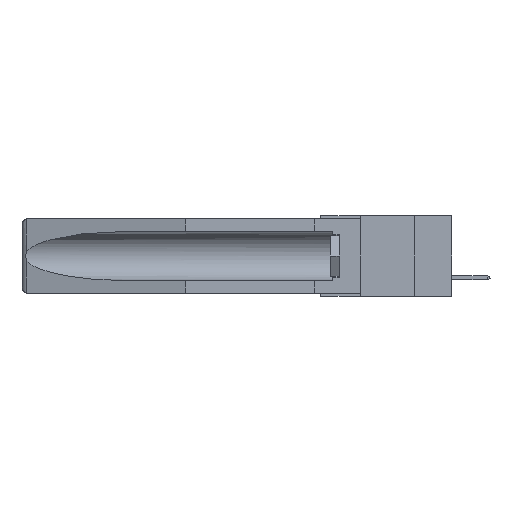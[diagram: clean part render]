
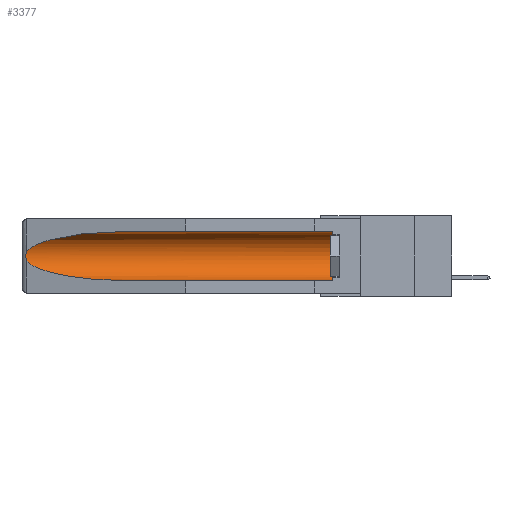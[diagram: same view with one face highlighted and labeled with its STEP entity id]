
A CAD part, left-side view. The second image highlights one B-rep face of the part: STEP entity #3377.
In plain terms, the highlighted cylindrical face has radius 2.857 mm (diameter 5.715 mm), a partial arc.
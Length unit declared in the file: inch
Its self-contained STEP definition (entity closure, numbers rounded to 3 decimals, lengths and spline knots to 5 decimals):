
#98 = EDGE_CURVE ( 'NONE', #11760, #6277, #2606, .T. ) ;
#481 = VERTEX_POINT ( 'NONE', #11869 ) ;
#518 = CARTESIAN_POINT ( 'NONE',  ( 0.155, -0.30754, -0.059 ) ) ;
#708 = VERTEX_POINT ( 'NONE', #5863 ) ;
#745 = CARTESIAN_POINT ( 'NONE',  ( 0.155, -0.30754, -0.1715 ) ) ;
#775 = ORIENTED_EDGE ( 'NONE', *, *, #9795, .T. ) ;
#1007 = EDGE_CURVE ( 'NONE', #2104, #481, #1783, .T. ) ;
#1044 = CARTESIAN_POINT ( 'NONE',  ( 0.26654, 1.53092, -0.15636 ) ) ;
#1214 = CARTESIAN_POINT ( 'NONE',  ( 0.26537, 1.52718, -0.19328 ) ) ;
#1607 = EDGE_LOOP ( 'NONE', ( #10839, #13551, #9595, #5077, #775, #15207 ) ) ;
#1783 = LINE ( 'NONE', #3878, #2586 ) ;
#2083 = CARTESIAN_POINT ( 'NONE',  ( 0.155, 1.07973, -0.059 ) ) ;
#2104 = VERTEX_POINT ( 'NONE', #11595 ) ;
#2303 = CARTESIAN_POINT ( 'NONE',  ( 0.26537, 1.52718, -0.14972 ) ) ;
#2393 = CARTESIAN_POINT ( 'NONE',  ( 0.2673, 1.53269, -0.17917 ) ) ;
#2586 = VECTOR ( 'NONE', #7704, 39.37008 ) ;
#2606 =( BOUNDED_CURVE ( )  B_SPLINE_CURVE ( 3, ( #13710, #8583, #14930, #11187 ),
 .UNSPECIFIED., .F., .F. ) 
 B_SPLINE_CURVE_WITH_KNOTS ( ( 4, 4 ),
 ( 4.71239, 6.08839 ),
 .UNSPECIFIED. ) 
 CURVE ( )  GEOMETRIC_REPRESENTATION_ITEM ( )  RATIONAL_B_SPLINE_CURVE ( ( 1., 0.848, 0.848, 1. ) ) 
 REPRESENTATION_ITEM ( '' )  );
#3377 = ADVANCED_FACE ( 'NONE', ( #11342 ), #6699, .F. ) ;
#3878 = CARTESIAN_POINT ( 'NONE',  ( 0.155, -0.30754, -0.284 ) ) ;
#4699 = CARTESIAN_POINT ( 'NONE',  ( 0.21114, 1.30732, -0.284 ) ) ;
#4751 = DIRECTION ( 'NONE',  ( 0., 1., 0. ) ) ;
#4930 = CARTESIAN_POINT ( 'NONE',  ( 0.2675, 1.53308, -0.17534 ) ) ;
#5051 = CARTESIAN_POINT ( 'NONE',  ( 0.26655, 1.53094, -0.18657 ) ) ;
#5077 = ORIENTED_EDGE ( 'NONE', *, *, #1007, .F. ) ;
#5108 = CARTESIAN_POINT ( 'NONE',  ( 0.2673, 1.5327, -0.16383 ) ) ;
#5169 = CARTESIAN_POINT ( 'NONE',  ( 0.26597, 1.52961, -0.15275 ) ) ;
#5863 = CARTESIAN_POINT ( 'NONE',  ( 0.26537, 1.52718, -0.19328 ) ) ;
#6277 = VERTEX_POINT ( 'NONE', #2303 ) ;
#6699 = CYLINDRICAL_SURFACE ( 'NONE', #14297, 0.1125 ) ;
#6906 = DIRECTION ( 'NONE',  ( 0., -1., 0. ) ) ;
#7704 = DIRECTION ( 'NONE',  ( 0., 1., 0. ) ) ;
#7753 = EDGE_CURVE ( 'NONE', #708, #481, #15104, .T. ) ;
#8543 = CARTESIAN_POINT ( 'NONE',  ( 0.26537, 1.52718, -0.19328 ) ) ;
#8583 = CARTESIAN_POINT ( 'NONE',  ( 0.21114, 1.30732, -0.059 ) ) ;
#8663 = CARTESIAN_POINT ( 'NONE',  ( 0.25451, 1.48313, -0.24835 ) ) ;
#9271 = DIRECTION ( 'NONE',  ( 0., 0., 1. ) ) ;
#9595 = ORIENTED_EDGE ( 'NONE', *, *, #7753, .T. ) ;
#9620 = DIRECTION ( 'NONE',  ( 0., 1., 0. ) ) ;
#9795 = EDGE_CURVE ( 'NONE', #2104, #12895, #16523, .T. ) ;
#10309 = CARTESIAN_POINT ( 'NONE',  ( 0.26597, 1.5296, -0.19026 ) ) ;
#10784 = CARTESIAN_POINT ( 'NONE',  ( 0.155, 0.126, -0.1715 ) ) ;
#10839 = ORIENTED_EDGE ( 'NONE', *, *, #98, .T. ) ;
#11187 = CARTESIAN_POINT ( 'NONE',  ( 0.26537, 1.52718, -0.14972 ) ) ;
#11342 = FACE_OUTER_BOUND ( 'NONE', #1607, .T. ) ;
#11595 = CARTESIAN_POINT ( 'NONE',  ( 0.155, 0.126, -0.284 ) ) ;
#11760 = VERTEX_POINT ( 'NONE', #2083 ) ;
#11869 = CARTESIAN_POINT ( 'NONE',  ( 0.155, 1.07973, -0.284 ) ) ;
#12346 = B_SPLINE_CURVE_WITH_KNOTS ( 'NONE', 3,
 ( #12692, #5169, #1044, #5108, #12806, #4930, #2393, #5051, #10309, #1214 ),
 .UNSPECIFIED., .F., .F.,
 ( 4, 2, 2, 2, 4 ),
 ( 0., 0.00029, 0.00058, 0.00087, 0.00117 ),
 .UNSPECIFIED. ) ;
#12399 = LINE ( 'NONE', #518, #15804 ) ;
#12692 = CARTESIAN_POINT ( 'NONE',  ( 0.26537, 1.52718, -0.14972 ) ) ;
#12806 = CARTESIAN_POINT ( 'NONE',  ( 0.2675, 1.53308, -0.16763 ) ) ;
#12895 = VERTEX_POINT ( 'NONE', #16528 ) ;
#13551 = ORIENTED_EDGE ( 'NONE', *, *, #13603, .T. ) ;
#13603 = EDGE_CURVE ( 'NONE', #6277, #708, #12346, .T. ) ;
#13710 = CARTESIAN_POINT ( 'NONE',  ( 0.155, 1.07973, -0.059 ) ) ;
#13836 = CARTESIAN_POINT ( 'NONE',  ( 0.155, 1.07973, -0.284 ) ) ;
#14297 = AXIS2_PLACEMENT_3D ( 'NONE', #745, #4751, #16351 ) ;
#14813 = EDGE_CURVE ( 'NONE', #12895, #11760, #12399, .T. ) ;
#14930 = CARTESIAN_POINT ( 'NONE',  ( 0.25451, 1.48313, -0.09465 ) ) ;
#15104 =( BOUNDED_CURVE ( )  B_SPLINE_CURVE ( 3, ( #8543, #8663, #4699, #13836 ),
 .UNSPECIFIED., .F., .F. ) 
 B_SPLINE_CURVE_WITH_KNOTS ( ( 4, 4 ),
 ( 0.1948, 1.5708 ),
 .UNSPECIFIED. ) 
 CURVE ( )  GEOMETRIC_REPRESENTATION_ITEM ( )  RATIONAL_B_SPLINE_CURVE ( ( 1., 0.848, 0.848, 1. ) ) 
 REPRESENTATION_ITEM ( '' )  );
#15207 = ORIENTED_EDGE ( 'NONE', *, *, #14813, .T. ) ;
#15804 = VECTOR ( 'NONE', #9620, 39.37008 ) ;
#16082 = AXIS2_PLACEMENT_3D ( 'NONE', #10784, #6906, #9271 ) ;
#16351 = DIRECTION ( 'NONE',  ( 0., 0., 1. ) ) ;
#16523 = CIRCLE ( 'NONE', #16082, 0.1125 ) ;
#16528 = CARTESIAN_POINT ( 'NONE',  ( 0.155, 0.126, -0.059 ) ) ;
